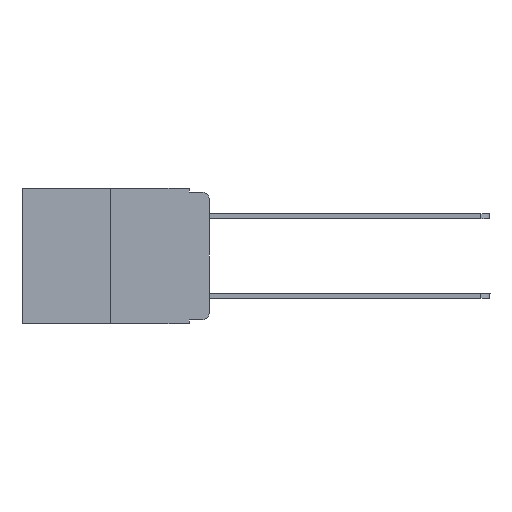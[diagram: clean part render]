
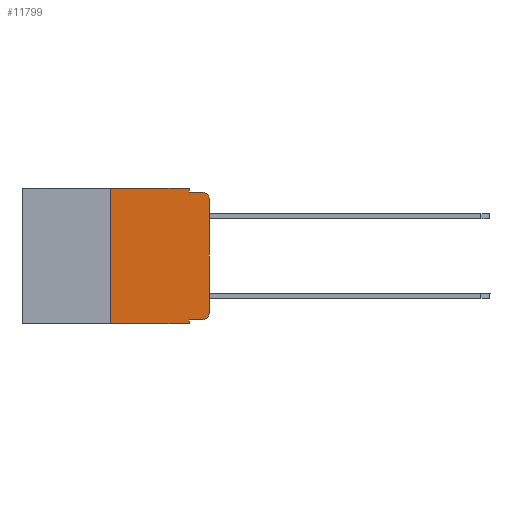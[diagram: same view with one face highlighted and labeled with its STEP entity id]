
A CAD part, left-side view. The second image highlights one B-rep face of the part: STEP entity #11799.
In plain terms, the highlighted planar face has unit normal (-1, 0, 0).
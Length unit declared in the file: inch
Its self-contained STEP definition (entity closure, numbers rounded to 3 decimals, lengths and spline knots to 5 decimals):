
#69 = ORIENTED_EDGE ( 'NONE', *, *, #7897, .T. ) ;
#827 = DIRECTION ( 'NONE',  ( 0., -1., 0. ) ) ;
#840 = CIRCLE ( 'NONE', #5499, 0.02 ) ;
#905 = CARTESIAN_POINT ( 'NONE',  ( 0., 0.473, -0.343 ) ) ;
#951 = EDGE_CURVE ( 'NONE', #3738, #7877, #9789, .T. ) ;
#1267 = CARTESIAN_POINT ( 'NONE',  ( 0., 0.051, -0.333 ) ) ;
#1419 = LINE ( 'NONE', #2880, #10116 ) ;
#1788 = VECTOR ( 'NONE', #827, 39.37008 ) ;
#1861 = ORIENTED_EDGE ( 'NONE', *, *, #10776, .F. ) ;
#1988 = VERTEX_POINT ( 'NONE', #10047 ) ;
#2051 = CARTESIAN_POINT ( 'NONE',  ( 0., 0.051, -0.333 ) ) ;
#2067 = DIRECTION ( 'NONE',  ( 0., 0., -1. ) ) ;
#2162 = EDGE_CURVE ( 'NONE', #13914, #7471, #11559, .T. ) ;
#2492 = CARTESIAN_POINT ( 'NONE',  ( 0., 0.02, -0.333 ) ) ;
#2753 = DIRECTION ( 'NONE',  ( 0., 0., -1. ) ) ;
#2806 = VERTEX_POINT ( 'NONE', #2492 ) ;
#2880 = CARTESIAN_POINT ( 'NONE',  ( 0., 0.051, 0. ) ) ;
#3142 = VECTOR ( 'NONE', #12021, 39.37008 ) ;
#3274 = ORIENTED_EDGE ( 'NONE', *, *, #2162, .F. ) ;
#3401 = CARTESIAN_POINT ( 'NONE',  ( 0., 0.02, -0.03 ) ) ;
#3471 = EDGE_CURVE ( 'NONE', #13404, #12045, #9804, .T. ) ;
#3527 = VERTEX_POINT ( 'NONE', #7383 ) ;
#3738 = VERTEX_POINT ( 'NONE', #11698 ) ;
#4236 = DIRECTION ( 'NONE',  ( 1., 0., 0. ) ) ;
#4311 = VECTOR ( 'NONE', #13031, 39.37008 ) ;
#4462 = VERTEX_POINT ( 'NONE', #7944 ) ;
#5279 = VECTOR ( 'NONE', #14671, 39.37008 ) ;
#5367 = CARTESIAN_POINT ( 'NONE',  ( 0., 0., 0. ) ) ;
#5464 = PLANE ( 'NONE',  #10100 ) ;
#5499 = AXIS2_PLACEMENT_3D ( 'NONE', #3401, #12635, #13938 ) ;
#5775 = CARTESIAN_POINT ( 'NONE',  ( 0., 0.051, 0. ) ) ;
#6236 = ORIENTED_EDGE ( 'NONE', *, *, #12623, .T. ) ;
#6391 = DIRECTION ( 'NONE',  ( 0., -1., 0. ) ) ;
#7383 = CARTESIAN_POINT ( 'NONE',  ( 0., 0.051, 0. ) ) ;
#7459 = CARTESIAN_POINT ( 'NONE',  ( 0., 0.051, -0.01 ) ) ;
#7471 = VERTEX_POINT ( 'NONE', #12651 ) ;
#7480 = CARTESIAN_POINT ( 'NONE',  ( 0., 0., -0.03 ) ) ;
#7733 = VECTOR ( 'NONE', #8822, 39.37008 ) ;
#7877 = VERTEX_POINT ( 'NONE', #7480 ) ;
#7897 = EDGE_CURVE ( 'NONE', #7877, #12045, #840, .T. ) ;
#7944 = CARTESIAN_POINT ( 'NONE',  ( 0., 0.25, 0. ) ) ;
#7948 = VECTOR ( 'NONE', #12298, 39.37008 ) ;
#8457 = LINE ( 'NONE', #14609, #7948 ) ;
#8822 = DIRECTION ( 'NONE',  ( 0., -1., 0. ) ) ;
#9571 = ORIENTED_EDGE ( 'NONE', *, *, #13401, .F. ) ;
#9603 = LINE ( 'NONE', #12876, #4311 ) ;
#9657 = EDGE_LOOP ( 'NONE', ( #10665, #69, #13256, #1861, #9571, #10052, #9697, #3274, #11453, #6236 ) ) ;
#9697 = ORIENTED_EDGE ( 'NONE', *, *, #10167, .T. ) ;
#9789 = LINE ( 'NONE', #5367, #5279 ) ;
#9804 = LINE ( 'NONE', #7459, #12672 ) ;
#10047 = CARTESIAN_POINT ( 'NONE',  ( 0., 0.25, -0.343 ) ) ;
#10052 = ORIENTED_EDGE ( 'NONE', *, *, #11209, .F. ) ;
#10100 = AXIS2_PLACEMENT_3D ( 'NONE', #14910, #4236, #2067 ) ;
#10116 = VECTOR ( 'NONE', #14494, 39.37008 ) ;
#10167 = EDGE_CURVE ( 'NONE', #1988, #7471, #11245, .T. ) ;
#10665 = ORIENTED_EDGE ( 'NONE', *, *, #951, .T. ) ;
#10776 = EDGE_CURVE ( 'NONE', #3527, #13404, #1419, .T. ) ;
#11102 = CARTESIAN_POINT ( 'NONE',  ( 0., 0.051, -0.01 ) ) ;
#11209 = EDGE_CURVE ( 'NONE', #1988, #4462, #8457, .T. ) ;
#11245 = LINE ( 'NONE', #905, #1788 ) ;
#11453 = ORIENTED_EDGE ( 'NONE', *, *, #13478, .T. ) ;
#11482 = FACE_OUTER_BOUND ( 'NONE', #9657, .T. ) ;
#11559 = LINE ( 'NONE', #5775, #3142 ) ;
#11636 = CARTESIAN_POINT ( 'NONE',  ( 0., 0.02, -0.01 ) ) ;
#11698 = CARTESIAN_POINT ( 'NONE',  ( 0., 0., -0.313 ) ) ;
#11799 = ADVANCED_FACE ( 'NONE', ( #11482 ), #5464, .F. ) ;
#11837 = CARTESIAN_POINT ( 'NONE',  ( 0., 0.02, -0.313 ) ) ;
#12021 = DIRECTION ( 'NONE',  ( 0., 0., -1. ) ) ;
#12045 = VERTEX_POINT ( 'NONE', #11636 ) ;
#12298 = DIRECTION ( 'NONE',  ( 0., 0., 1. ) ) ;
#12317 = CIRCLE ( 'NONE', #14761, 0.02 ) ;
#12623 = EDGE_CURVE ( 'NONE', #2806, #3738, #12317, .T. ) ;
#12635 = DIRECTION ( 'NONE',  ( -1., 0., 0. ) ) ;
#12651 = CARTESIAN_POINT ( 'NONE',  ( 0., 0.051, -0.343 ) ) ;
#12672 = VECTOR ( 'NONE', #6391, 39.37008 ) ;
#12876 = CARTESIAN_POINT ( 'NONE',  ( 0., 0.473, 0. ) ) ;
#13031 = DIRECTION ( 'NONE',  ( 0., -1., 0. ) ) ;
#13236 = DIRECTION ( 'NONE',  ( -1., 0., 0. ) ) ;
#13256 = ORIENTED_EDGE ( 'NONE', *, *, #3471, .F. ) ;
#13401 = EDGE_CURVE ( 'NONE', #4462, #3527, #9603, .T. ) ;
#13404 = VERTEX_POINT ( 'NONE', #11102 ) ;
#13478 = EDGE_CURVE ( 'NONE', #13914, #2806, #14684, .T. ) ;
#13914 = VERTEX_POINT ( 'NONE', #1267 ) ;
#13938 = DIRECTION ( 'NONE',  ( 0., 0., -1. ) ) ;
#14494 = DIRECTION ( 'NONE',  ( 0., 0., -1. ) ) ;
#14609 = CARTESIAN_POINT ( 'NONE',  ( 0., 0.25, 0. ) ) ;
#14671 = DIRECTION ( 'NONE',  ( 0., 0., 1. ) ) ;
#14684 = LINE ( 'NONE', #2051, #7733 ) ;
#14761 = AXIS2_PLACEMENT_3D ( 'NONE', #11837, #13236, #2753 ) ;
#14910 = CARTESIAN_POINT ( 'NONE',  ( 0., 0.473, 0. ) ) ;
